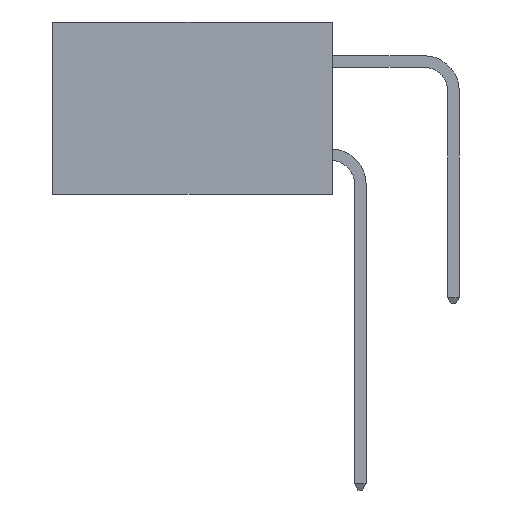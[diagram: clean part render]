
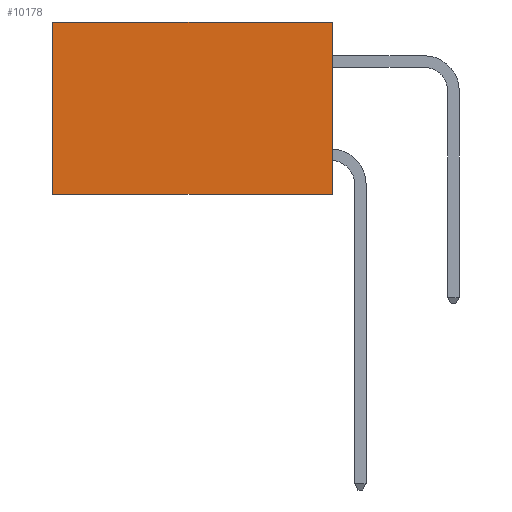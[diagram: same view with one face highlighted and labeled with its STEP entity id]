
A CAD part, left-side view. The second image highlights one B-rep face of the part: STEP entity #10178.
In plain terms, the highlighted planar face has unit normal (-1, 0, 0).
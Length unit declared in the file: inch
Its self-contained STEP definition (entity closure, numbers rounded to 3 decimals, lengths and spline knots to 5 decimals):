
#578 = CARTESIAN_POINT ( 'NONE',  ( 0.2615, 0., 0. ) ) ;
#1054 = CARTESIAN_POINT ( 'NONE',  ( 0.2615, 0.6, -0.37 ) ) ;
#1400 = VECTOR ( 'NONE', #18651, 39.37008 ) ;
#2030 = VERTEX_POINT ( 'NONE', #7533 ) ;
#3749 = ORIENTED_EDGE ( 'NONE', *, *, #11326, .T. ) ;
#3869 = CARTESIAN_POINT ( 'NONE',  ( 0.2615, 0.6, -0.37 ) ) ;
#4491 = VECTOR ( 'NONE', #11130, 39.37008 ) ;
#5575 = LINE ( 'NONE', #1054, #1400 ) ;
#6847 = CARTESIAN_POINT ( 'NONE',  ( 0.2615, 0., -0.37 ) ) ;
#7384 = EDGE_CURVE ( 'NONE', #2030, #12047, #5575, .T. ) ;
#7423 = VECTOR ( 'NONE', #14226, 39.37008 ) ;
#7533 = CARTESIAN_POINT ( 'NONE',  ( 0.2615, 0.6, 0. ) ) ;
#7901 = LINE ( 'NONE', #9662, #7423 ) ;
#8290 = LINE ( 'NONE', #6847, #15869 ) ;
#9098 = CARTESIAN_POINT ( 'NONE',  ( 0.2615, 0., -0.37 ) ) ;
#9586 = CARTESIAN_POINT ( 'NONE',  ( 0.2615, 0., 0. ) ) ;
#9662 = CARTESIAN_POINT ( 'NONE',  ( 0.2615, 0., -0.37 ) ) ;
#10178 = ADVANCED_FACE ( 'NONE', ( #16872 ), #10393, .F. ) ;
#10292 = DIRECTION ( 'NONE',  ( 0., 0., -1. ) ) ;
#10393 = PLANE ( 'NONE',  #14165 ) ;
#10482 = CARTESIAN_POINT ( 'NONE',  ( 0.2615, 0., -0.37 ) ) ;
#11130 = DIRECTION ( 'NONE',  ( 0., 1., 0. ) ) ;
#11326 = EDGE_CURVE ( 'NONE', #13352, #2030, #13527, .T. ) ;
#12018 = EDGE_CURVE ( 'NONE', #13352, #12321, #8290, .T. ) ;
#12047 = VERTEX_POINT ( 'NONE', #3869 ) ;
#12321 = VERTEX_POINT ( 'NONE', #9098 ) ;
#13245 = DIRECTION ( 'NONE',  ( 1., 0., 0. ) ) ;
#13352 = VERTEX_POINT ( 'NONE', #578 ) ;
#13527 = LINE ( 'NONE', #9586, #4491 ) ;
#13906 = ORIENTED_EDGE ( 'NONE', *, *, #12018, .F. ) ;
#14165 = AXIS2_PLACEMENT_3D ( 'NONE', #10482, #13245, #10292 ) ;
#14226 = DIRECTION ( 'NONE',  ( 0., 1., 0. ) ) ;
#15232 = EDGE_LOOP ( 'NONE', ( #19325, #15259, #13906, #3749 ) ) ;
#15259 = ORIENTED_EDGE ( 'NONE', *, *, #15675, .F. ) ;
#15675 = EDGE_CURVE ( 'NONE', #12321, #12047, #7901, .T. ) ;
#15869 = VECTOR ( 'NONE', #17452, 39.37008 ) ;
#16872 = FACE_OUTER_BOUND ( 'NONE', #15232, .T. ) ;
#17452 = DIRECTION ( 'NONE',  ( 0., 0., -1. ) ) ;
#18651 = DIRECTION ( 'NONE',  ( 0., 0., -1. ) ) ;
#19325 = ORIENTED_EDGE ( 'NONE', *, *, #7384, .T. ) ;
